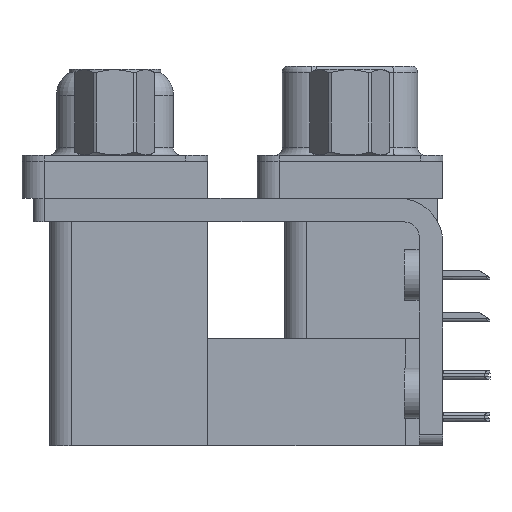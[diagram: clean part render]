
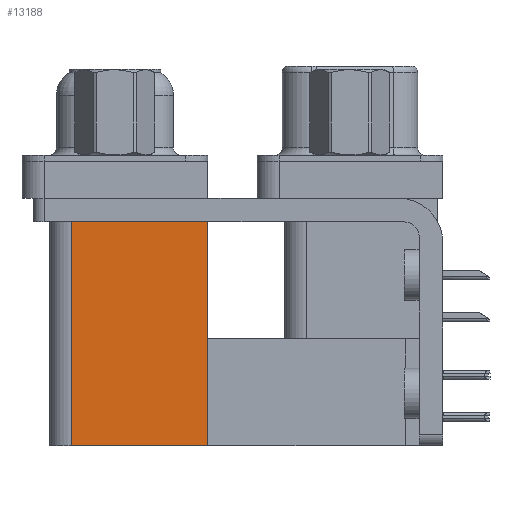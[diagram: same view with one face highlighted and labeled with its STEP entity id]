
A CAD part, left-side view. The second image highlights one B-rep face of the part: STEP entity #13188.
In plain terms, the highlighted planar face has unit normal (-1, 0, 0).
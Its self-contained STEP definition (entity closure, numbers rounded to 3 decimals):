
#94 = DIRECTION ( 'NONE',  ( 1., 0., 0. ) ) ;
#348 = VERTEX_POINT ( 'NONE', #33644 ) ;
#411 = CARTESIAN_POINT ( 'NONE',  ( 3.765, 9.6, -19.2 ) ) ;
#788 = CARTESIAN_POINT ( 'NONE',  ( 3.765, 18.8, -19.2 ) ) ;
#2305 = EDGE_CURVE ( 'NONE', #20398, #23363, #51335, .T. ) ;
#3048 = VERTEX_POINT ( 'NONE', #23744 ) ;
#3259 = VECTOR ( 'NONE', #31350, 1000. ) ;
#3879 = LINE ( 'NONE', #35292, #25272 ) ;
#4530 = ORIENTED_EDGE ( 'NONE', *, *, #30263, .T. ) ;
#8536 = ORIENTED_EDGE ( 'NONE', *, *, #36944, .T. ) ;
#8922 = DIRECTION ( 'NONE',  ( 0., 0., -1. ) ) ;
#10939 = LINE ( 'NONE', #22838, #21106 ) ;
#13188 = ADVANCED_FACE ( 'NONE', ( #36397 ), #44210, .F. ) ;
#13480 = CARTESIAN_POINT ( 'NONE',  ( 3.765, 18.8, -2.5 ) ) ;
#15044 = VECTOR ( 'NONE', #28446, 1000. ) ;
#15287 = CARTESIAN_POINT ( 'NONE',  ( 3.765, 18.8, -19.2 ) ) ;
#18445 = DIRECTION ( 'NONE',  ( 0., 0., 1. ) ) ;
#19714 = DIRECTION ( 'NONE',  ( 0., 1., 0. ) ) ;
#20398 = VERTEX_POINT ( 'NONE', #788 ) ;
#21106 = VECTOR ( 'NONE', #18445, 1000. ) ;
#22379 = ORIENTED_EDGE ( 'NONE', *, *, #2305, .F. ) ;
#22838 = CARTESIAN_POINT ( 'NONE',  ( 3.765, 9.6, -19.2 ) ) ;
#23363 = VERTEX_POINT ( 'NONE', #13480 ) ;
#23744 = CARTESIAN_POINT ( 'NONE',  ( 3.765, 9.6, -19.2 ) ) ;
#25145 = EDGE_CURVE ( 'NONE', #3048, #20398, #46110, .T. ) ;
#25272 = VECTOR ( 'NONE', #19714, 1000. ) ;
#28446 = DIRECTION ( 'NONE',  ( 0., 1., 0. ) ) ;
#30263 = EDGE_CURVE ( 'NONE', #348, #23363, #3879, .T. ) ;
#30388 = ORIENTED_EDGE ( 'NONE', *, *, #25145, .F. ) ;
#31350 = DIRECTION ( 'NONE',  ( 0., 0., 1. ) ) ;
#33644 = CARTESIAN_POINT ( 'NONE',  ( 3.765, 9.6, -2.5 ) ) ;
#35292 = CARTESIAN_POINT ( 'NONE',  ( 3.765, 9.6, -2.5 ) ) ;
#36397 = FACE_OUTER_BOUND ( 'NONE', #50373, .T. ) ;
#36944 = EDGE_CURVE ( 'NONE', #3048, #348, #10939, .T. ) ;
#42849 = AXIS2_PLACEMENT_3D ( 'NONE', #43955, #94, #8922 ) ;
#43955 = CARTESIAN_POINT ( 'NONE',  ( 3.765, 9.6, -19.2 ) ) ;
#44210 = PLANE ( 'NONE',  #42849 ) ;
#46110 = LINE ( 'NONE', #411, #15044 ) ;
#50373 = EDGE_LOOP ( 'NONE', ( #4530, #22379, #30388, #8536 ) ) ;
#51335 = LINE ( 'NONE', #15287, #3259 ) ;
